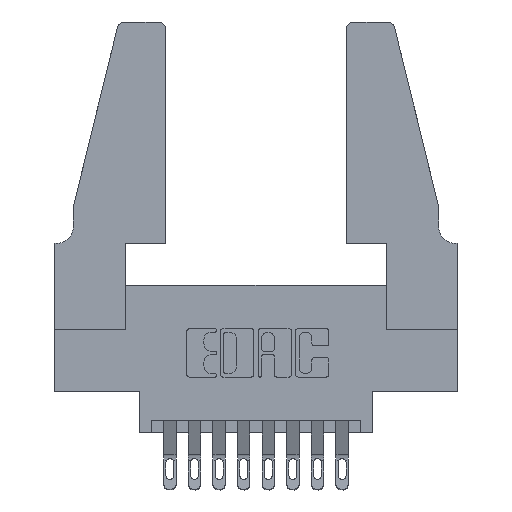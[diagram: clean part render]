
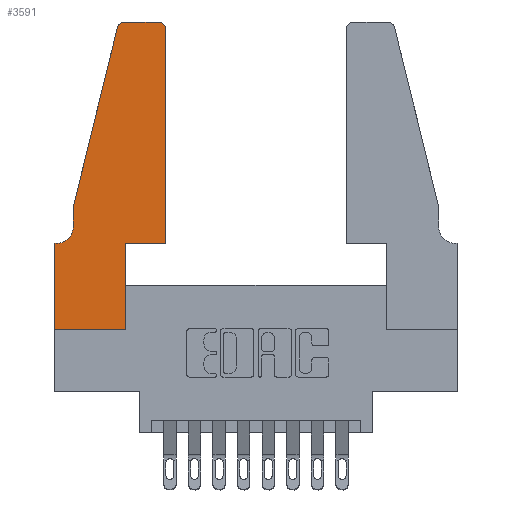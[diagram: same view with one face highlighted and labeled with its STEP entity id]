
A CAD part, top view. The second image highlights one B-rep face of the part: STEP entity #3591.
In plain terms, the highlighted planar face has unit normal (0, 0, 1).
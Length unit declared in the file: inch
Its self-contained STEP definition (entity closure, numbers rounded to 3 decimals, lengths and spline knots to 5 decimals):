
#31 = ORIENTED_EDGE ( 'NONE', *, *, #8390, .T. ) ;
#32 = VECTOR ( 'NONE', #7798, 39.37008 ) ;
#102 = LINE ( 'NONE', #10618, #10567 ) ;
#244 = CARTESIAN_POINT ( 'NONE',  ( 0., 0.35, 0.37 ) ) ;
#408 = LINE ( 'NONE', #6752, #32 ) ;
#423 = FACE_OUTER_BOUND ( 'NONE', #5931, .T. ) ;
#439 = AXIS2_PLACEMENT_3D ( 'NONE', #9496, #3276, #10533 ) ;
#746 = VERTEX_POINT ( 'NONE', #1697 ) ;
#868 = VERTEX_POINT ( 'NONE', #244 ) ;
#947 = DIRECTION ( 'NONE',  ( 1., 0., 0. ) ) ;
#1016 = CARTESIAN_POINT ( 'NONE',  ( 0.4505, 0.35, 0.37 ) ) ;
#1065 = CARTESIAN_POINT ( 'NONE',  ( 0.2865, 0.35, 0.37 ) ) ;
#1237 = EDGE_CURVE ( 'NONE', #12433, #12071, #10270, .T. ) ;
#1248 = CARTESIAN_POINT ( 'NONE',  ( 0.4505, 0.35, 0.37 ) ) ;
#1379 = ORIENTED_EDGE ( 'NONE', *, *, #8462, .T. ) ;
#1440 = VECTOR ( 'NONE', #8444, 39.37008 ) ;
#1579 = CARTESIAN_POINT ( 'NONE',  ( 0.0755, 0.5, 0.37 ) ) ;
#1646 = VECTOR ( 'NONE', #12746, 39.37008 ) ;
#1697 = CARTESIAN_POINT ( 'NONE',  ( 0.2865, 0., 0.37 ) ) ;
#1720 = DIRECTION ( 'NONE',  ( 1., 0., 0. ) ) ;
#1748 = VERTEX_POINT ( 'NONE', #6857 ) ;
#1766 = ORIENTED_EDGE ( 'NONE', *, *, #6740, .T. ) ;
#2108 = EDGE_CURVE ( 'NONE', #1748, #6286, #9914, .T. ) ;
#2473 = VECTOR ( 'NONE', #8385, 39.37008 ) ;
#2586 = VERTEX_POINT ( 'NONE', #13426 ) ;
#2969 = DIRECTION ( 'NONE',  ( -1., 0., 0. ) ) ;
#3049 = CARTESIAN_POINT ( 'NONE',  ( 0.0755, 0.42, 0.37 ) ) ;
#3107 = EDGE_CURVE ( 'NONE', #2586, #868, #3702, .T. ) ;
#3276 = DIRECTION ( 'NONE',  ( 0., 0., -1. ) ) ;
#3294 = CARTESIAN_POINT ( 'NONE',  ( 0.2605, 1.25, 0.37 ) ) ;
#3356 = DIRECTION ( 'NONE',  ( -0.239, -0.971, 0. ) ) ;
#3370 = ORIENTED_EDGE ( 'NONE', *, *, #3107, .T. ) ;
#3527 = LINE ( 'NONE', #5875, #12702 ) ;
#3591 = ADVANCED_FACE ( 'NONE', ( #423 ), #9828, .T. ) ;
#3702 = LINE ( 'NONE', #10115, #9241 ) ;
#3886 = DIRECTION ( 'NONE',  ( -1., 0., 0. ) ) ;
#3892 = ORIENTED_EDGE ( 'NONE', *, *, #9651, .T. ) ;
#4122 = EDGE_CURVE ( 'NONE', #4135, #4488, #408, .T. ) ;
#4135 = VERTEX_POINT ( 'NONE', #8837 ) ;
#4287 = LINE ( 'NONE', #1248, #6737 ) ;
#4488 = VERTEX_POINT ( 'NONE', #1016 ) ;
#4829 = CIRCLE ( 'NONE', #13324, 0.03 ) ;
#5073 = EDGE_CURVE ( 'NONE', #6731, #1748, #4829, .T. ) ;
#5165 = CARTESIAN_POINT ( 'NONE',  ( 0., 0., 0.37 ) ) ;
#5222 = ORIENTED_EDGE ( 'NONE', *, *, #13360, .T. ) ;
#5424 = CARTESIAN_POINT ( 'NONE',  ( 0.4505, 1.22, 0.37 ) ) ;
#5725 = DIRECTION ( 'NONE',  ( 0., 0., 1. ) ) ;
#5875 = CARTESIAN_POINT ( 'NONE',  ( 0., 0., 0.37 ) ) ;
#5931 = EDGE_LOOP ( 'NONE', ( #9840, #5222, #1379, #9875, #31, #3370, #3892, #11654, #12943, #6360, #1766, #11832 ) ) ;
#6083 = AXIS2_PLACEMENT_3D ( 'NONE', #11878, #5725, #12898 ) ;
#6216 = CARTESIAN_POINT ( 'NONE',  ( 0.284, 1.22, 0.37 ) ) ;
#6286 = VERTEX_POINT ( 'NONE', #6800 ) ;
#6353 = CARTESIAN_POINT ( 'NONE',  ( 0., 0., 0.37 ) ) ;
#6360 = ORIENTED_EDGE ( 'NONE', *, *, #4122, .T. ) ;
#6653 = EDGE_CURVE ( 'NONE', #746, #4135, #11076, .T. ) ;
#6731 = VERTEX_POINT ( 'NONE', #5424 ) ;
#6737 = VECTOR ( 'NONE', #12592, 39.37008 ) ;
#6740 = EDGE_CURVE ( 'NONE', #4488, #6731, #4287, .T. ) ;
#6752 = CARTESIAN_POINT ( 'NONE',  ( 0.4505, 0.35, 0.37 ) ) ;
#6800 = CARTESIAN_POINT ( 'NONE',  ( 0.284, 1.25, 0.37 ) ) ;
#6809 = AXIS2_PLACEMENT_3D ( 'NONE', #6216, #13403, #7276 ) ;
#6857 = CARTESIAN_POINT ( 'NONE',  ( 0.4205, 1.25, 0.37 ) ) ;
#7001 = LINE ( 'NONE', #6353, #1440 ) ;
#7184 = VECTOR ( 'NONE', #2969, 39.37008 ) ;
#7239 = DIRECTION ( 'NONE',  ( 0., 0., 1. ) ) ;
#7276 = DIRECTION ( 'NONE',  ( 1., 0., 0. ) ) ;
#7798 = DIRECTION ( 'NONE',  ( 1., 0., 0. ) ) ;
#8385 = DIRECTION ( 'NONE',  ( 0., 1., 0. ) ) ;
#8390 = EDGE_CURVE ( 'NONE', #12071, #2586, #11215, .T. ) ;
#8444 = DIRECTION ( 'NONE',  ( 0., -1., 0. ) ) ;
#8462 = EDGE_CURVE ( 'NONE', #10773, #12433, #102, .T. ) ;
#8837 = CARTESIAN_POINT ( 'NONE',  ( 0.2865, 0.35, 0.37 ) ) ;
#9241 = VECTOR ( 'NONE', #3886, 39.37008 ) ;
#9496 = CARTESIAN_POINT ( 'NONE',  ( 0.0055, 0.42, 0.37 ) ) ;
#9651 = EDGE_CURVE ( 'NONE', #868, #12091, #7001, .T. ) ;
#9828 = PLANE ( 'NONE',  #6083 ) ;
#9840 = ORIENTED_EDGE ( 'NONE', *, *, #2108, .T. ) ;
#9875 = ORIENTED_EDGE ( 'NONE', *, *, #1237, .T. ) ;
#9914 = LINE ( 'NONE', #3294, #7184 ) ;
#10115 = CARTESIAN_POINT ( 'NONE',  ( 0.0755, 0.35, 0.37 ) ) ;
#10270 = LINE ( 'NONE', #12933, #1646 ) ;
#10301 = CARTESIAN_POINT ( 'NONE',  ( 0.25487, 1.22718, 0.37 ) ) ;
#10533 = DIRECTION ( 'NONE',  ( -1., 0., 0. ) ) ;
#10567 = VECTOR ( 'NONE', #3356, 39.37008 ) ;
#10616 = EDGE_CURVE ( 'NONE', #12091, #746, #3527, .T. ) ;
#10618 = CARTESIAN_POINT ( 'NONE',  ( 0.0755, 0.5, 0.37 ) ) ;
#10773 = VERTEX_POINT ( 'NONE', #10301 ) ;
#11076 = LINE ( 'NONE', #1065, #2473 ) ;
#11215 = CIRCLE ( 'NONE', #439, 0.07 ) ;
#11654 = ORIENTED_EDGE ( 'NONE', *, *, #10616, .T. ) ;
#11832 = ORIENTED_EDGE ( 'NONE', *, *, #5073, .T. ) ;
#11878 = CARTESIAN_POINT ( 'NONE',  ( 0., 0.35, 0.37 ) ) ;
#11998 = CIRCLE ( 'NONE', #6809, 0.03 ) ;
#12071 = VERTEX_POINT ( 'NONE', #3049 ) ;
#12091 = VERTEX_POINT ( 'NONE', #5165 ) ;
#12433 = VERTEX_POINT ( 'NONE', #1579 ) ;
#12592 = DIRECTION ( 'NONE',  ( 0., 1., 0. ) ) ;
#12702 = VECTOR ( 'NONE', #1720, 39.37008 ) ;
#12746 = DIRECTION ( 'NONE',  ( 0., -1., 0. ) ) ;
#12898 = DIRECTION ( 'NONE',  ( 1., 0., 0. ) ) ;
#12933 = CARTESIAN_POINT ( 'NONE',  ( 0.0755, 0.5, 0.37 ) ) ;
#12943 = ORIENTED_EDGE ( 'NONE', *, *, #6653, .T. ) ;
#13324 = AXIS2_PLACEMENT_3D ( 'NONE', #13368, #7239, #947 ) ;
#13360 = EDGE_CURVE ( 'NONE', #6286, #10773, #11998, .T. ) ;
#13368 = CARTESIAN_POINT ( 'NONE',  ( 0.4205, 1.22, 0.37 ) ) ;
#13403 = DIRECTION ( 'NONE',  ( 0., 0., 1. ) ) ;
#13426 = CARTESIAN_POINT ( 'NONE',  ( 0.0055, 0.35, 0.37 ) ) ;
